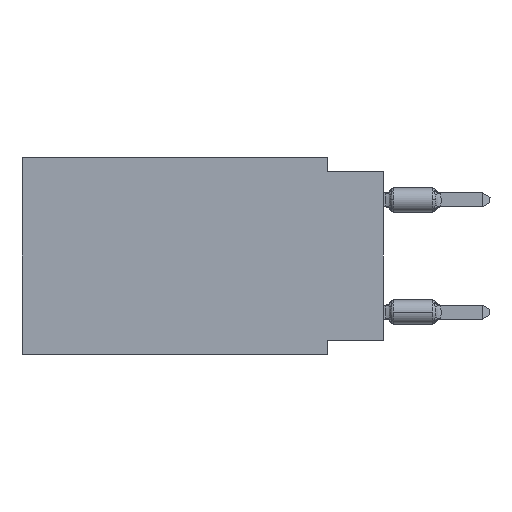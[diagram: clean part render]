
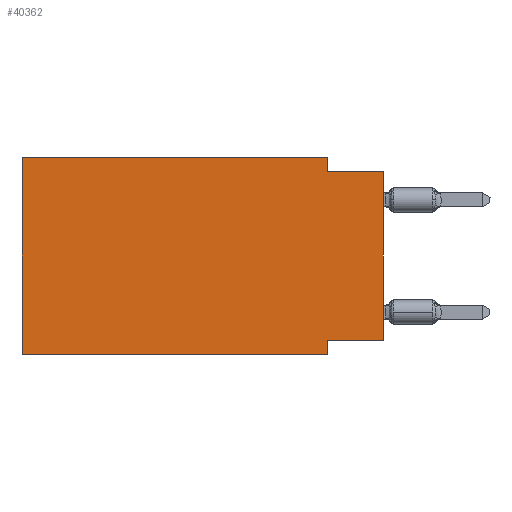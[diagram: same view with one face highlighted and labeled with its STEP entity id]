
A CAD part, left-side view. The second image highlights one B-rep face of the part: STEP entity #40362.
In plain terms, the highlighted planar face has unit normal (-1, 0, 0).
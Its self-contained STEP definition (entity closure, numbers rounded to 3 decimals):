
#308 = DIRECTION ( 'NONE',  ( 0., -1., 0. ) ) ;
#2272 = DIRECTION ( 'NONE',  ( 0., 0., 1. ) ) ;
#2522 = LINE ( 'NONE', #54423, #24121 ) ;
#2885 = EDGE_CURVE ( 'NONE', #8841, #11838, #55994, .T. ) ;
#3046 = CARTESIAN_POINT ( 'NONE',  ( 0., 16.383, 0. ) ) ;
#3415 = EDGE_CURVE ( 'NONE', #47929, #45771, #5456, .T. ) ;
#3587 = LINE ( 'NONE', #55176, #5803 ) ;
#3909 = ORIENTED_EDGE ( 'NONE', *, *, #26984, .F. ) ;
#3950 = EDGE_CURVE ( 'NONE', #12537, #36908, #16237, .T. ) ;
#4947 = CARTESIAN_POINT ( 'NONE',  ( 0., 16.383, 0. ) ) ;
#5456 = LINE ( 'NONE', #53321, #55798 ) ;
#5803 = VECTOR ( 'NONE', #41504, 1000. ) ;
#6154 = EDGE_CURVE ( 'NONE', #12537, #45771, #37620, .T. ) ;
#6271 = VERTEX_POINT ( 'NONE', #20486 ) ;
#7170 = ORIENTED_EDGE ( 'NONE', *, *, #7603, .T. ) ;
#7409 = VERTEX_POINT ( 'NONE', #9954 ) ;
#7535 = ORIENTED_EDGE ( 'NONE', *, *, #2885, .F. ) ;
#7603 = EDGE_CURVE ( 'NONE', #6271, #7409, #45983, .T. ) ;
#7746 = DIRECTION ( 'NONE',  ( 0., 0., 1. ) ) ;
#8841 = VERTEX_POINT ( 'NONE', #25481 ) ;
#9621 = LINE ( 'NONE', #24214, #33736 ) ;
#9954 = CARTESIAN_POINT ( 'NONE',  ( 0., 0., -0.635 ) ) ;
#10101 = VECTOR ( 'NONE', #28927, 1000. ) ;
#11768 = ORIENTED_EDGE ( 'NONE', *, *, #38616, .F. ) ;
#11794 = CARTESIAN_POINT ( 'NONE',  ( 0., 0., 0. ) ) ;
#11838 = VERTEX_POINT ( 'NONE', #35720 ) ;
#12537 = VERTEX_POINT ( 'NONE', #20578 ) ;
#13410 = CARTESIAN_POINT ( 'NONE',  ( 0., 2.54, 0. ) ) ;
#13916 = ORIENTED_EDGE ( 'NONE', *, *, #17817, .F. ) ;
#16237 = LINE ( 'NONE', #26493, #43956 ) ;
#17817 = EDGE_CURVE ( 'NONE', #36908, #8841, #2522, .T. ) ;
#20486 = CARTESIAN_POINT ( 'NONE',  ( 0., 0., -8.255 ) ) ;
#20578 = CARTESIAN_POINT ( 'NONE',  ( 0., 16.383, -8.89 ) ) ;
#22377 = ORIENTED_EDGE ( 'NONE', *, *, #3415, .F. ) ;
#24121 = VECTOR ( 'NONE', #41899, 1000. ) ;
#24214 = CARTESIAN_POINT ( 'NONE',  ( 0., 0., -0.635 ) ) ;
#25481 = CARTESIAN_POINT ( 'NONE',  ( 0., 2.54, 0. ) ) ;
#25924 = AXIS2_PLACEMENT_3D ( 'NONE', #4947, #38515, #57459 ) ;
#26493 = CARTESIAN_POINT ( 'NONE',  ( 0., 16.383, 0. ) ) ;
#26984 = EDGE_CURVE ( 'NONE', #11838, #7409, #9621, .T. ) ;
#27599 = EDGE_LOOP ( 'NONE', ( #7170, #3909, #7535, #13916, #29634, #46642, #22377, #11768 ) ) ;
#28927 = DIRECTION ( 'NONE',  ( 0., 0., -1. ) ) ;
#29634 = ORIENTED_EDGE ( 'NONE', *, *, #3950, .F. ) ;
#31728 = CARTESIAN_POINT ( 'NONE',  ( 0., 2.54, -8.255 ) ) ;
#33231 = FACE_OUTER_BOUND ( 'NONE', #27599, .T. ) ;
#33736 = VECTOR ( 'NONE', #308, 1000. ) ;
#35720 = CARTESIAN_POINT ( 'NONE',  ( 0., 2.54, -0.635 ) ) ;
#36706 = DIRECTION ( 'NONE',  ( 0., -1., 0. ) ) ;
#36908 = VERTEX_POINT ( 'NONE', #3046 ) ;
#37016 = CARTESIAN_POINT ( 'NONE',  ( 0., 16.383, -8.89 ) ) ;
#37620 = LINE ( 'NONE', #37016, #41032 ) ;
#38204 = PLANE ( 'NONE',  #25924 ) ;
#38515 = DIRECTION ( 'NONE',  ( 1., 0., 0. ) ) ;
#38616 = EDGE_CURVE ( 'NONE', #6271, #47929, #3587, .T. ) ;
#40130 = VECTOR ( 'NONE', #7746, 1000. ) ;
#40362 = ADVANCED_FACE ( 'NONE', ( #33231 ), #38204, .F. ) ;
#41032 = VECTOR ( 'NONE', #36706, 1000. ) ;
#41504 = DIRECTION ( 'NONE',  ( 0., 1., 0. ) ) ;
#41899 = DIRECTION ( 'NONE',  ( 0., -1., 0. ) ) ;
#43956 = VECTOR ( 'NONE', #2272, 1000. ) ;
#44082 = CARTESIAN_POINT ( 'NONE',  ( 0., 2.54, -8.89 ) ) ;
#45771 = VERTEX_POINT ( 'NONE', #44082 ) ;
#45983 = LINE ( 'NONE', #11794, #40130 ) ;
#46642 = ORIENTED_EDGE ( 'NONE', *, *, #6154, .T. ) ;
#47929 = VERTEX_POINT ( 'NONE', #31728 ) ;
#48960 = DIRECTION ( 'NONE',  ( 0., 0., -1. ) ) ;
#53321 = CARTESIAN_POINT ( 'NONE',  ( 0., 2.54, -8.89 ) ) ;
#54423 = CARTESIAN_POINT ( 'NONE',  ( 0., 16.383, 0. ) ) ;
#55176 = CARTESIAN_POINT ( 'NONE',  ( 0., 0., -8.255 ) ) ;
#55798 = VECTOR ( 'NONE', #48960, 1000. ) ;
#55994 = LINE ( 'NONE', #13410, #10101 ) ;
#57459 = DIRECTION ( 'NONE',  ( 0., 0., -1. ) ) ;
